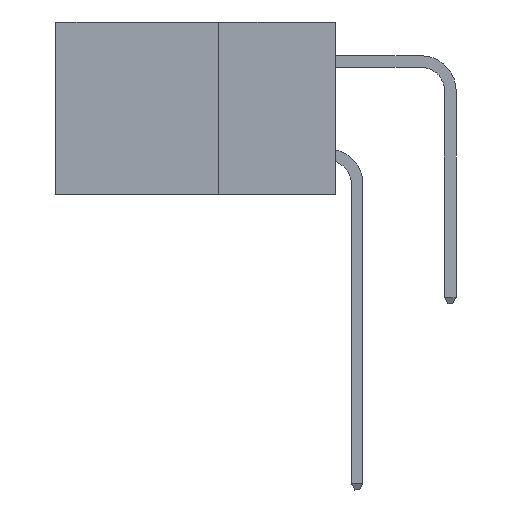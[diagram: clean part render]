
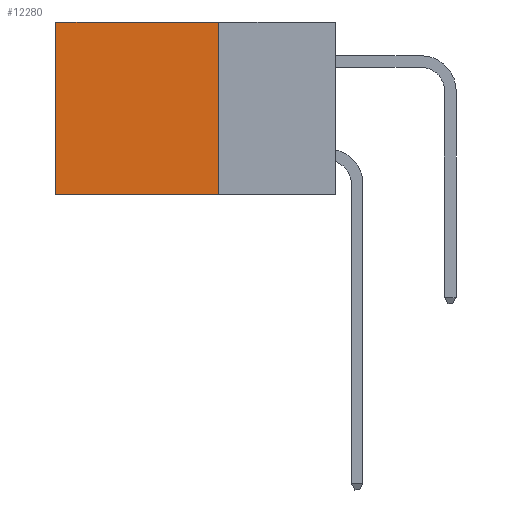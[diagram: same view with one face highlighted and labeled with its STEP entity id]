
A CAD part, left-side view. The second image highlights one B-rep face of the part: STEP entity #12280.
In plain terms, the highlighted planar face has unit normal (-1, 0, 0).
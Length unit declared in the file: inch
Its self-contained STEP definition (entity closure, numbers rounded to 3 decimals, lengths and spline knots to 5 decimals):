
#453 = CARTESIAN_POINT ( 'NONE',  ( 0.2875, 0.25, 0. ) ) ;
#1439 = EDGE_LOOP ( 'NONE', ( #15401, #3512, #7117, #6920 ) ) ;
#1734 = EDGE_CURVE ( 'NONE', #9421, #10063, #16716, .T. ) ;
#2864 = EDGE_CURVE ( 'NONE', #13353, #10063, #9358, .T. ) ;
#2935 = CARTESIAN_POINT ( 'NONE',  ( 0.2875, 0.25, -0.37 ) ) ;
#2982 = CARTESIAN_POINT ( 'NONE',  ( 0.2875, 0.6, 0. ) ) ;
#3409 = DIRECTION ( 'NONE',  ( 0., 1., 0. ) ) ;
#3512 = ORIENTED_EDGE ( 'NONE', *, *, #1734, .F. ) ;
#4483 = DIRECTION ( 'NONE',  ( 0., 0., -1. ) ) ;
#4874 = VECTOR ( 'NONE', #4483, 39.37008 ) ;
#5421 = DIRECTION ( 'NONE',  ( 0., 0., -1. ) ) ;
#6371 = CARTESIAN_POINT ( 'NONE',  ( 0.2875, 0.25, 0. ) ) ;
#6920 = ORIENTED_EDGE ( 'NONE', *, *, #8453, .T. ) ;
#7117 = ORIENTED_EDGE ( 'NONE', *, *, #12948, .F. ) ;
#7921 = DIRECTION ( 'NONE',  ( 0., 0., -1. ) ) ;
#8453 = EDGE_CURVE ( 'NONE', #14062, #13353, #18529, .T. ) ;
#8875 = VECTOR ( 'NONE', #5421, 39.37008 ) ;
#8990 = CARTESIAN_POINT ( 'NONE',  ( 0.2875, 0.6, -0.37 ) ) ;
#9212 = DIRECTION ( 'NONE',  ( 0., 1., 0. ) ) ;
#9358 = LINE ( 'NONE', #2982, #4874 ) ;
#9421 = VERTEX_POINT ( 'NONE', #2935 ) ;
#9791 = LINE ( 'NONE', #12716, #8875 ) ;
#10026 = FACE_OUTER_BOUND ( 'NONE', #1439, .T. ) ;
#10063 = VERTEX_POINT ( 'NONE', #8990 ) ;
#12223 = CARTESIAN_POINT ( 'NONE',  ( 0.2875, 0.6, 0. ) ) ;
#12280 = ADVANCED_FACE ( 'NONE', ( #10026 ), #15034, .F. ) ;
#12716 = CARTESIAN_POINT ( 'NONE',  ( 0.2875, 0.25, 0. ) ) ;
#12948 = EDGE_CURVE ( 'NONE', #14062, #9421, #9791, .T. ) ;
#12952 = VECTOR ( 'NONE', #9212, 39.37008 ) ;
#13308 = AXIS2_PLACEMENT_3D ( 'NONE', #6371, #16443, #7921 ) ;
#13353 = VERTEX_POINT ( 'NONE', #12223 ) ;
#13672 = CARTESIAN_POINT ( 'NONE',  ( 0.2875, 0.25, 0. ) ) ;
#14062 = VERTEX_POINT ( 'NONE', #453 ) ;
#15034 = PLANE ( 'NONE',  #13308 ) ;
#15237 = VECTOR ( 'NONE', #3409, 39.37008 ) ;
#15401 = ORIENTED_EDGE ( 'NONE', *, *, #2864, .T. ) ;
#16443 = DIRECTION ( 'NONE',  ( 1., 0., 0. ) ) ;
#16716 = LINE ( 'NONE', #17700, #12952 ) ;
#17700 = CARTESIAN_POINT ( 'NONE',  ( 0.2875, 0.25, -0.37 ) ) ;
#18529 = LINE ( 'NONE', #13672, #15237 ) ;
